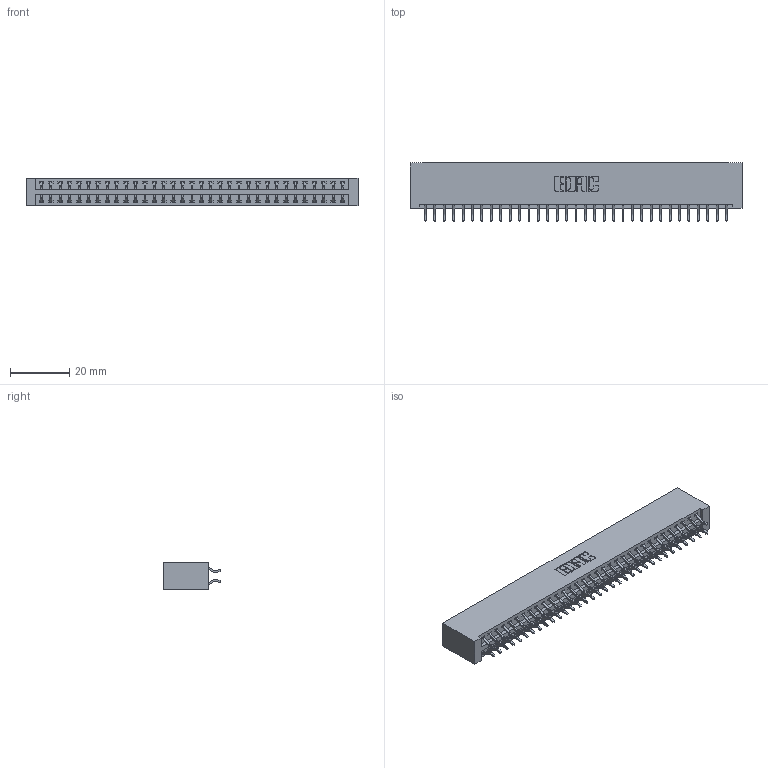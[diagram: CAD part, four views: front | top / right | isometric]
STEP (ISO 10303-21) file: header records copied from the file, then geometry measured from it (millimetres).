
FILE_DESCRIPTION (( 'STEP AP203' ), '1' );
FILE_NAME ('346-066-556-201.STEP', '2022-05-24T17:43:33', ( '' ), ( '' ), 'SwSTEP 2.0', 'SolidWorks 2020', '' );
FILE_SCHEMA (( 'CONFIG_CONTROL_DESIGN' ));
Length unit declared in the file: inch
Products named in the file (3): 346 Part_No Mounting Lugs; 345-292-001_556 Tail; 346-066-556-201
Assembly tree (67 placements, depth 2):
  346-066-556-201
    346 Part_No Mounting Lugs
    345-292-001_556 Tail  x66
Bounding box: 112.01 x 19.57 x 9.4 mm (x, y, z)
Volume: 11423.5 mm3; surface area: 15662.8 mm2
Topology: 67 solids, 67 shells, 3942 faces, 11723 edges, 7726 vertices
Faces by surface type: plane 2646, cylinder 1296
Entity records: 22691 total; most frequent: CARTESIAN_POINT 3764, ORIENTED_EDGE 3686, DIRECTION 3351, EDGE_CURVE 1843, LINE 1579, VECTOR 1579, VERTEX_POINT 1226, AXIS2_PLACEMENT_3D 886
